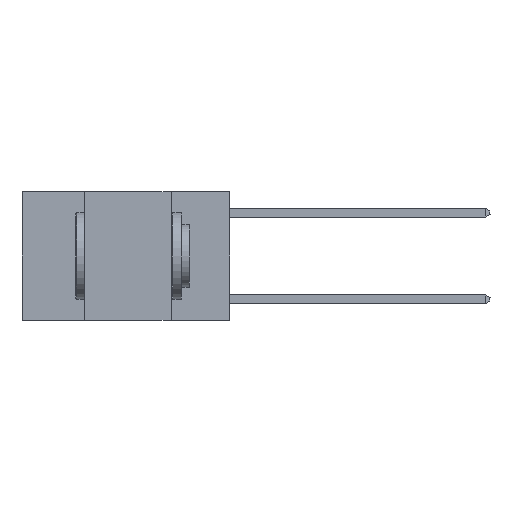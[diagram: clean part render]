
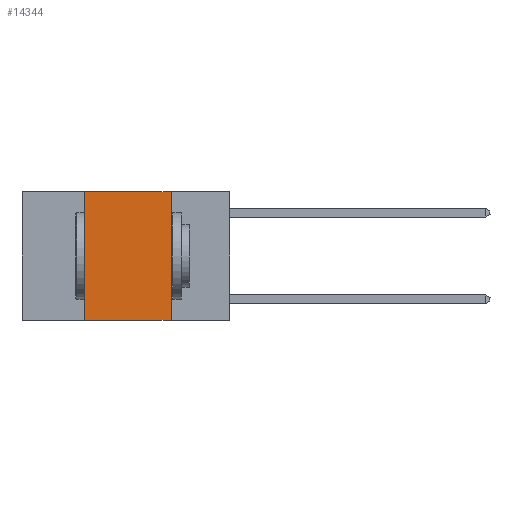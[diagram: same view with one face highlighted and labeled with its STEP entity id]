
A CAD part, left-side view. The second image highlights one B-rep face of the part: STEP entity #14344.
In plain terms, the highlighted planar face has unit normal (-1, 0, 0).
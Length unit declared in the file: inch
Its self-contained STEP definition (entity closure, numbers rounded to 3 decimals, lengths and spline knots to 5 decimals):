
#1720 = CARTESIAN_POINT ( 'NONE',  ( 0., 0.42, -0.37 ) ) ;
#1851 = LINE ( 'NONE', #9671, #3008 ) ;
#1915 = CARTESIAN_POINT ( 'NONE',  ( 0., 0.17, 0. ) ) ;
#2233 = EDGE_CURVE ( 'NONE', #17767, #6681, #1851, .T. ) ;
#2317 = ORIENTED_EDGE ( 'NONE', *, *, #2233, .F. ) ;
#3008 = VECTOR ( 'NONE', #17323, 39.37008 ) ;
#3119 = AXIS2_PLACEMENT_3D ( 'NONE', #19355, #5565, #8181 ) ;
#3205 = EDGE_CURVE ( 'NONE', #6681, #16835, #9529, .T. ) ;
#4913 = CARTESIAN_POINT ( 'NONE',  ( 0., 0.17, -0.37 ) ) ;
#5077 = DIRECTION ( 'NONE',  ( 0., -1., 0. ) ) ;
#5565 = DIRECTION ( 'NONE',  ( 1., 0., 0. ) ) ;
#6199 = LINE ( 'NONE', #6400, #15327 ) ;
#6400 = CARTESIAN_POINT ( 'NONE',  ( 0., 0.6, -0.37 ) ) ;
#6681 = VERTEX_POINT ( 'NONE', #17113 ) ;
#7628 = VECTOR ( 'NONE', #9696, 39.37008 ) ;
#8181 = DIRECTION ( 'NONE',  ( 0., 0., -1. ) ) ;
#8497 = ORIENTED_EDGE ( 'NONE', *, *, #15457, .F. ) ;
#9340 = DIRECTION ( 'NONE',  ( 0., 0., -1. ) ) ;
#9529 = LINE ( 'NONE', #1915, #14626 ) ;
#9599 = CARTESIAN_POINT ( 'NONE',  ( 0., 0.42, 0. ) ) ;
#9671 = CARTESIAN_POINT ( 'NONE',  ( 0., 0.6, 0. ) ) ;
#9696 = DIRECTION ( 'NONE',  ( 0., 0., 1. ) ) ;
#12792 = CARTESIAN_POINT ( 'NONE',  ( 0., 0.42, 0. ) ) ;
#13114 = FACE_OUTER_BOUND ( 'NONE', #17028, .T. ) ;
#13204 = PLANE ( 'NONE',  #3119 ) ;
#14153 = EDGE_CURVE ( 'NONE', #16248, #16835, #6199, .T. ) ;
#14344 = ADVANCED_FACE ( 'NONE', ( #13114 ), #13204, .F. ) ;
#14626 = VECTOR ( 'NONE', #9340, 39.37008 ) ;
#15327 = VECTOR ( 'NONE', #5077, 39.37008 ) ;
#15457 = EDGE_CURVE ( 'NONE', #16248, #17767, #16780, .T. ) ;
#16248 = VERTEX_POINT ( 'NONE', #1720 ) ;
#16780 = LINE ( 'NONE', #9599, #7628 ) ;
#16835 = VERTEX_POINT ( 'NONE', #4913 ) ;
#17028 = EDGE_LOOP ( 'NONE', ( #19599, #2317, #8497, #19322 ) ) ;
#17113 = CARTESIAN_POINT ( 'NONE',  ( 0., 0.17, 0. ) ) ;
#17323 = DIRECTION ( 'NONE',  ( 0., -1., 0. ) ) ;
#17767 = VERTEX_POINT ( 'NONE', #12792 ) ;
#19322 = ORIENTED_EDGE ( 'NONE', *, *, #14153, .T. ) ;
#19355 = CARTESIAN_POINT ( 'NONE',  ( 0., 0.6, 0. ) ) ;
#19599 = ORIENTED_EDGE ( 'NONE', *, *, #3205, .F. ) ;
